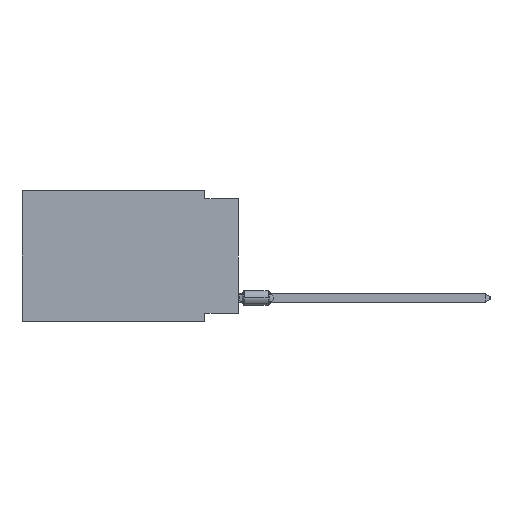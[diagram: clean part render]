
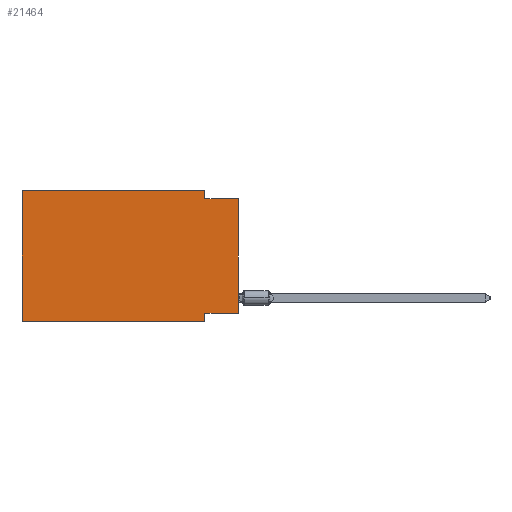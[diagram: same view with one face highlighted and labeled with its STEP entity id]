
A CAD part, left-side view. The second image highlights one B-rep face of the part: STEP entity #21464.
In plain terms, the highlighted planar face has unit normal (-1, 0, 0).
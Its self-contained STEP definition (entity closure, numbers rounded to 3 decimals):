
#788 = FACE_OUTER_BOUND ( 'NONE', #33806, .T. ) ;
#2480 = VERTEX_POINT ( 'NONE', #12883 ) ;
#2706 = LINE ( 'NONE', #55524, #27689 ) ;
#2899 = CARTESIAN_POINT ( 'NONE',  ( 0., 16.383, 0. ) ) ;
#3331 = AXIS2_PLACEMENT_3D ( 'NONE', #4297, #13702, #18377 ) ;
#3696 = LINE ( 'NONE', #11646, #21812 ) ;
#4297 = CARTESIAN_POINT ( 'NONE',  ( 0., 16.383, 0. ) ) ;
#6057 = EDGE_CURVE ( 'NONE', #50382, #37319, #27204, .T. ) ;
#7868 = VECTOR ( 'NONE', #18741, 1000. ) ;
#9018 = CARTESIAN_POINT ( 'NONE',  ( 0., 0., -0.635 ) ) ;
#9955 = DIRECTION ( 'NONE',  ( 0., -1., 0. ) ) ;
#10609 = VERTEX_POINT ( 'NONE', #53540 ) ;
#11646 = CARTESIAN_POINT ( 'NONE',  ( 0., 2.54, 0. ) ) ;
#12485 = VECTOR ( 'NONE', #29007, 1000. ) ;
#12883 = CARTESIAN_POINT ( 'NONE',  ( 0., 2.54, -9.271 ) ) ;
#13410 = PLANE ( 'NONE',  #3331 ) ;
#13702 = DIRECTION ( 'NONE',  ( 1., 0., 0. ) ) ;
#13840 = VECTOR ( 'NONE', #26914, 1000. ) ;
#14067 = LINE ( 'NONE', #22865, #7868 ) ;
#16453 = ORIENTED_EDGE ( 'NONE', *, *, #29530, .F. ) ;
#16561 = EDGE_CURVE ( 'NONE', #10609, #43863, #51309, .T. ) ;
#18328 = ORIENTED_EDGE ( 'NONE', *, *, #16561, .F. ) ;
#18377 = DIRECTION ( 'NONE',  ( 0., 0., -1. ) ) ;
#18741 = DIRECTION ( 'NONE',  ( 0., 1., 0. ) ) ;
#19429 = ORIENTED_EDGE ( 'NONE', *, *, #50230, .T. ) ;
#19757 = EDGE_CURVE ( 'NONE', #30830, #2480, #14067, .T. ) ;
#20592 = DIRECTION ( 'NONE',  ( 0., 0., 1. ) ) ;
#21464 = ADVANCED_FACE ( 'NONE', ( #788 ), #13410, .F. ) ;
#21532 = VECTOR ( 'NONE', #41718, 1000. ) ;
#21812 = VECTOR ( 'NONE', #38611, 1000. ) ;
#21986 = CARTESIAN_POINT ( 'NONE',  ( 0., 16.383, -9.906 ) ) ;
#22865 = CARTESIAN_POINT ( 'NONE',  ( 0., 0., -9.271 ) ) ;
#23504 = EDGE_CURVE ( 'NONE', #27648, #50757, #40473, .T. ) ;
#23676 = ORIENTED_EDGE ( 'NONE', *, *, #32024, .F. ) ;
#26914 = DIRECTION ( 'NONE',  ( 0., -1., 0. ) ) ;
#27204 = LINE ( 'NONE', #9018, #13840 ) ;
#27648 = VERTEX_POINT ( 'NONE', #21986 ) ;
#27689 = VECTOR ( 'NONE', #20592, 1000. ) ;
#28211 = CARTESIAN_POINT ( 'NONE',  ( 0., 0., 0. ) ) ;
#29007 = DIRECTION ( 'NONE',  ( 0., -1., 0. ) ) ;
#29530 = EDGE_CURVE ( 'NONE', #2480, #50757, #34141, .T. ) ;
#30830 = VERTEX_POINT ( 'NONE', #30912 ) ;
#30912 = CARTESIAN_POINT ( 'NONE',  ( 0., 0., -9.271 ) ) ;
#31975 = VECTOR ( 'NONE', #43824, 1000. ) ;
#32024 = EDGE_CURVE ( 'NONE', #43863, #50382, #3696, .T. ) ;
#33806 = EDGE_LOOP ( 'NONE', ( #19429, #52688, #23676, #18328, #47105, #53092, #16453, #51101 ) ) ;
#34141 = LINE ( 'NONE', #52043, #31975 ) ;
#35063 = CARTESIAN_POINT ( 'NONE',  ( 0., 0., -0.635 ) ) ;
#37319 = VERTEX_POINT ( 'NONE', #35063 ) ;
#37596 = LINE ( 'NONE', #28211, #21532 ) ;
#38611 = DIRECTION ( 'NONE',  ( 0., 0., -1. ) ) ;
#40421 = CARTESIAN_POINT ( 'NONE',  ( 0., 2.54, 0. ) ) ;
#40473 = LINE ( 'NONE', #50708, #43892 ) ;
#41718 = DIRECTION ( 'NONE',  ( 0., 0., 1. ) ) ;
#43824 = DIRECTION ( 'NONE',  ( 0., 0., -1. ) ) ;
#43863 = VERTEX_POINT ( 'NONE', #40421 ) ;
#43892 = VECTOR ( 'NONE', #9955, 1000. ) ;
#45496 = EDGE_CURVE ( 'NONE', #27648, #10609, #2706, .T. ) ;
#47105 = ORIENTED_EDGE ( 'NONE', *, *, #45496, .F. ) ;
#48267 = CARTESIAN_POINT ( 'NONE',  ( 0., 2.54, -9.906 ) ) ;
#50001 = CARTESIAN_POINT ( 'NONE',  ( 0., 2.54, -0.635 ) ) ;
#50230 = EDGE_CURVE ( 'NONE', #30830, #37319, #37596, .T. ) ;
#50382 = VERTEX_POINT ( 'NONE', #50001 ) ;
#50708 = CARTESIAN_POINT ( 'NONE',  ( 0., 16.383, -9.906 ) ) ;
#50757 = VERTEX_POINT ( 'NONE', #48267 ) ;
#51101 = ORIENTED_EDGE ( 'NONE', *, *, #19757, .F. ) ;
#51309 = LINE ( 'NONE', #2899, #12485 ) ;
#52043 = CARTESIAN_POINT ( 'NONE',  ( 0., 2.54, -9.906 ) ) ;
#52688 = ORIENTED_EDGE ( 'NONE', *, *, #6057, .F. ) ;
#53092 = ORIENTED_EDGE ( 'NONE', *, *, #23504, .T. ) ;
#53540 = CARTESIAN_POINT ( 'NONE',  ( 0., 16.383, 0. ) ) ;
#55524 = CARTESIAN_POINT ( 'NONE',  ( 0., 16.383, 0. ) ) ;
